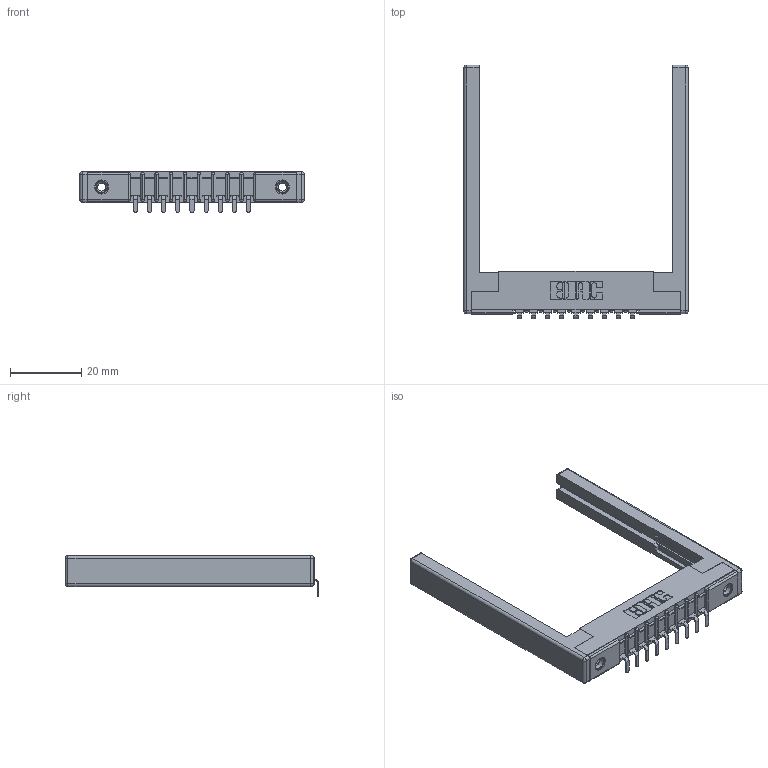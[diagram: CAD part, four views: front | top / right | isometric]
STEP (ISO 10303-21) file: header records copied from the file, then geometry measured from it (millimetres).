
FILE_DESCRIPTION (( 'STEP AP203' ), '1' );
FILE_NAME ('307-009-553-168.STEP', '2019-09-04T18:53:02', ( '' ), ( '' ), 'SwSTEP 2.0', 'SolidWorks 2016', '' );
FILE_SCHEMA (( 'CONFIG_CONTROL_DESIGN' ));
Length unit declared in the file: inch
Products named in the file (5): 307-290-002_553; 307 Part_.156 Dia Mounting Holes; 307-220-068; 307-009-553-168; 345-250-001_345-250-001-102
Assembly tree (14 placements, depth 2):
  307-009-553-168
    307 Part_.156 Dia Mounting Holes
    307-290-002_553  x9
    307-220-068  x2
    345-250-001_345-250-001-102  x2
Bounding box: 63.09 x 71.29 x 11.51 mm (x, y, z)
Volume: 8717.3 mm3; surface area: 10864 mm2
Topology: 14 solids, 14 shells, 984 faces, 2909 edges, 1890 vertices
Faces by surface type: plane 581, cylinder 359, sphere 28, cone 12, torus 4
Entity records: 15397 total; most frequent: CARTESIAN_POINT 2557, ORIENTED_EDGE 2536, DIRECTION 2518, EDGE_CURVE 1268, LINE 952, VECTOR 952, VERTEX_POINT 822, AXIS2_PLACEMENT_3D 783
